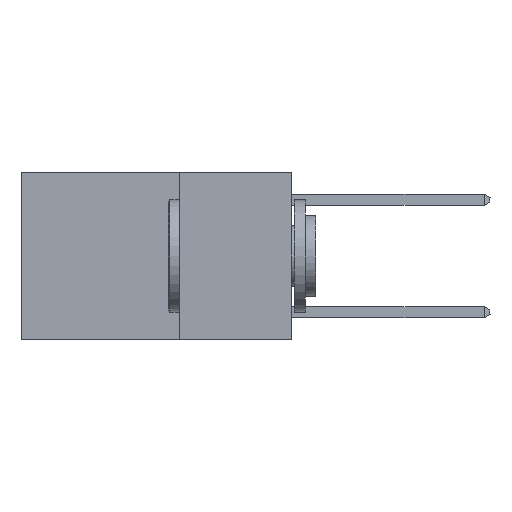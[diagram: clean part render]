
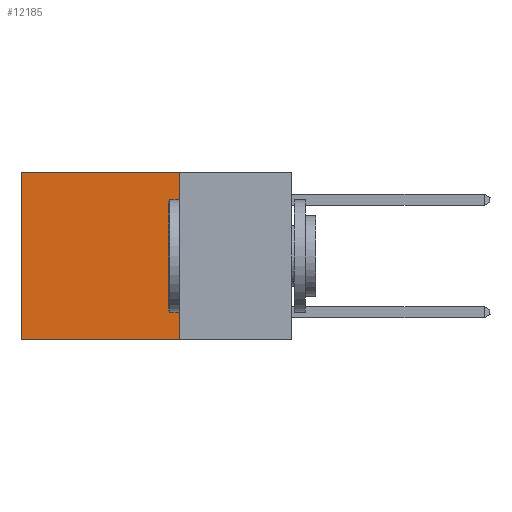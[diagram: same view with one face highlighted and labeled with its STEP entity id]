
A CAD part, left-side view. The second image highlights one B-rep face of the part: STEP entity #12185.
In plain terms, the highlighted planar face has unit normal (-1, 0, 0).
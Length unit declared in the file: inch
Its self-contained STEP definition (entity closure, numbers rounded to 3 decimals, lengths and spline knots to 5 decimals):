
#138 = CARTESIAN_POINT ( 'NONE',  ( 0.2625, 0.6, -0.37 ) ) ;
#1491 = LINE ( 'NONE', #13845, #12917 ) ;
#2074 = ORIENTED_EDGE ( 'NONE', *, *, #24195, .T. ) ;
#2362 = VERTEX_POINT ( 'NONE', #15021 ) ;
#3007 = CARTESIAN_POINT ( 'NONE',  ( 0.2625, 0.25, -0.37 ) ) ;
#3044 = AXIS2_PLACEMENT_3D ( 'NONE', #17222, #5149, #24937 ) ;
#3484 = VECTOR ( 'NONE', #20147, 39.37008 ) ;
#4939 = DIRECTION ( 'NONE',  ( 0., 1., 0. ) ) ;
#5149 = DIRECTION ( 'NONE',  ( 1., 0., 0. ) ) ;
#6093 = VECTOR ( 'NONE', #13725, 39.37008 ) ;
#7653 = LINE ( 'NONE', #10707, #20827 ) ;
#8962 = FACE_OUTER_BOUND ( 'NONE', #18096, .T. ) ;
#10184 = LINE ( 'NONE', #16364, #3484 ) ;
#10707 = CARTESIAN_POINT ( 'NONE',  ( 0.2625, 0.25, 0. ) ) ;
#12185 = ADVANCED_FACE ( 'NONE', ( #8962 ), #16972, .F. ) ;
#12917 = VECTOR ( 'NONE', #15700, 39.37008 ) ;
#13725 = DIRECTION ( 'NONE',  ( 0., 0., -1. ) ) ;
#13845 = CARTESIAN_POINT ( 'NONE',  ( 0.2625, 0.25, 0. ) ) ;
#14487 = EDGE_CURVE ( 'NONE', #2362, #16399, #17797, .T. ) ;
#15021 = CARTESIAN_POINT ( 'NONE',  ( 0.2625, 0.6, 0. ) ) ;
#15153 = ORIENTED_EDGE ( 'NONE', *, *, #17478, .F. ) ;
#15275 = VERTEX_POINT ( 'NONE', #3007 ) ;
#15700 = DIRECTION ( 'NONE',  ( 0., 0., -1. ) ) ;
#16081 = VERTEX_POINT ( 'NONE', #24978 ) ;
#16364 = CARTESIAN_POINT ( 'NONE',  ( 0.2625, 0.25, -0.37 ) ) ;
#16399 = VERTEX_POINT ( 'NONE', #138 ) ;
#16972 = PLANE ( 'NONE',  #3044 ) ;
#17222 = CARTESIAN_POINT ( 'NONE',  ( 0.2625, 0.25, 0. ) ) ;
#17478 = EDGE_CURVE ( 'NONE', #15275, #16399, #10184, .T. ) ;
#17550 = CARTESIAN_POINT ( 'NONE',  ( 0.2625, 0.6, 0. ) ) ;
#17797 = LINE ( 'NONE', #17550, #6093 ) ;
#18096 = EDGE_LOOP ( 'NONE', ( #22708, #15153, #22215, #2074 ) ) ;
#20147 = DIRECTION ( 'NONE',  ( 0., 1., 0. ) ) ;
#20827 = VECTOR ( 'NONE', #4939, 39.37008 ) ;
#22215 = ORIENTED_EDGE ( 'NONE', *, *, #25682, .F. ) ;
#22708 = ORIENTED_EDGE ( 'NONE', *, *, #14487, .T. ) ;
#24195 = EDGE_CURVE ( 'NONE', #16081, #2362, #7653, .T. ) ;
#24937 = DIRECTION ( 'NONE',  ( 0., 0., -1. ) ) ;
#24978 = CARTESIAN_POINT ( 'NONE',  ( 0.2625, 0.25, 0. ) ) ;
#25682 = EDGE_CURVE ( 'NONE', #16081, #15275, #1491, .T. ) ;
